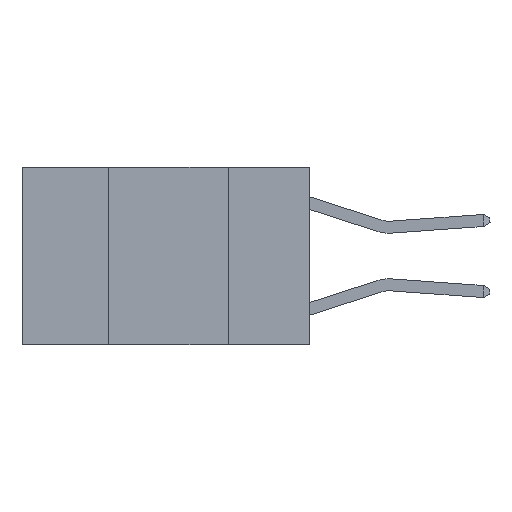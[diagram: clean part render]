
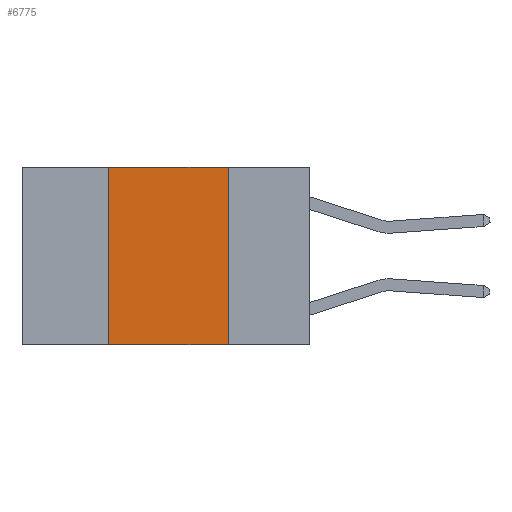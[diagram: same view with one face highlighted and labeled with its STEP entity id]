
A CAD part, left-side view. The second image highlights one B-rep face of the part: STEP entity #6775.
In plain terms, the highlighted planar face has unit normal (-1, 0, 0).
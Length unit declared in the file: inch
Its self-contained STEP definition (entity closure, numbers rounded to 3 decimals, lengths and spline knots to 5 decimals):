
#2227 = LINE ( 'NONE', #2815, #9484 ) ;
#2641 = VECTOR ( 'NONE', #3300, 39.37008 ) ;
#2815 = CARTESIAN_POINT ( 'NONE',  ( 0., 0.17, 0. ) ) ;
#3300 = DIRECTION ( 'NONE',  ( 0., -1., 0. ) ) ;
#4519 = LINE ( 'NONE', #13837, #26915 ) ;
#4834 = AXIS2_PLACEMENT_3D ( 'NONE', #11936, #23818, #12224 ) ;
#5722 = CARTESIAN_POINT ( 'NONE',  ( 0., 0.17, -0.37 ) ) ;
#6775 = ADVANCED_FACE ( 'NONE', ( #12081 ), #7489, .F. ) ;
#7489 = PLANE ( 'NONE',  #4834 ) ;
#7995 = EDGE_CURVE ( 'NONE', #8742, #20767, #10733, .T. ) ;
#8666 = CARTESIAN_POINT ( 'NONE',  ( 0., 0.42, 0. ) ) ;
#8742 = VERTEX_POINT ( 'NONE', #28372 ) ;
#9484 = VECTOR ( 'NONE', #18392, 39.37008 ) ;
#10593 = EDGE_CURVE ( 'NONE', #20767, #26696, #4519, .T. ) ;
#10703 = VERTEX_POINT ( 'NONE', #5722 ) ;
#10733 = LINE ( 'NONE', #20622, #13706 ) ;
#11936 = CARTESIAN_POINT ( 'NONE',  ( 0., 0.6, 0. ) ) ;
#12081 = FACE_OUTER_BOUND ( 'NONE', #14077, .T. ) ;
#12224 = DIRECTION ( 'NONE',  ( 0., 0., -1. ) ) ;
#12661 = ORIENTED_EDGE ( 'NONE', *, *, #10593, .F. ) ;
#13169 = EDGE_CURVE ( 'NONE', #8742, #10703, #16455, .T. ) ;
#13557 = EDGE_CURVE ( 'NONE', #26696, #10703, #2227, .T. ) ;
#13706 = VECTOR ( 'NONE', #22475, 39.37008 ) ;
#13837 = CARTESIAN_POINT ( 'NONE',  ( 0., 0.6, 0. ) ) ;
#14077 = EDGE_LOOP ( 'NONE', ( #29661, #12661, #24256, #16907 ) ) ;
#16455 = LINE ( 'NONE', #25751, #2641 ) ;
#16907 = ORIENTED_EDGE ( 'NONE', *, *, #13169, .T. ) ;
#18392 = DIRECTION ( 'NONE',  ( 0., 0., -1. ) ) ;
#20622 = CARTESIAN_POINT ( 'NONE',  ( 0., 0.42, 0. ) ) ;
#20767 = VERTEX_POINT ( 'NONE', #8666 ) ;
#21914 = DIRECTION ( 'NONE',  ( 0., -1., 0. ) ) ;
#22475 = DIRECTION ( 'NONE',  ( 0., 0., 1. ) ) ;
#22667 = CARTESIAN_POINT ( 'NONE',  ( 0., 0.17, 0. ) ) ;
#23818 = DIRECTION ( 'NONE',  ( 1., 0., 0. ) ) ;
#24256 = ORIENTED_EDGE ( 'NONE', *, *, #7995, .F. ) ;
#25751 = CARTESIAN_POINT ( 'NONE',  ( 0., 0.6, -0.37 ) ) ;
#26696 = VERTEX_POINT ( 'NONE', #22667 ) ;
#26915 = VECTOR ( 'NONE', #21914, 39.37008 ) ;
#28372 = CARTESIAN_POINT ( 'NONE',  ( 0., 0.42, -0.37 ) ) ;
#29661 = ORIENTED_EDGE ( 'NONE', *, *, #13557, .F. ) ;
